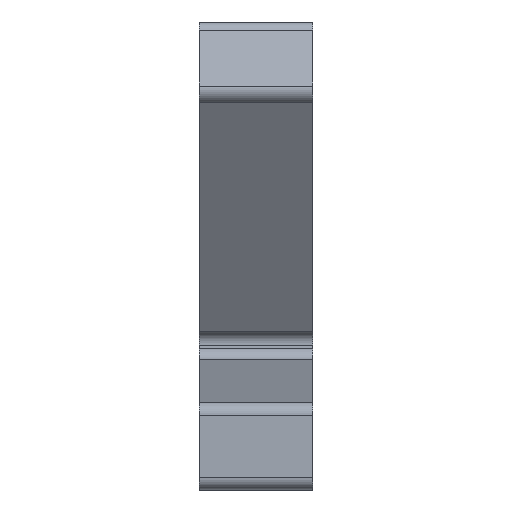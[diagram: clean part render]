
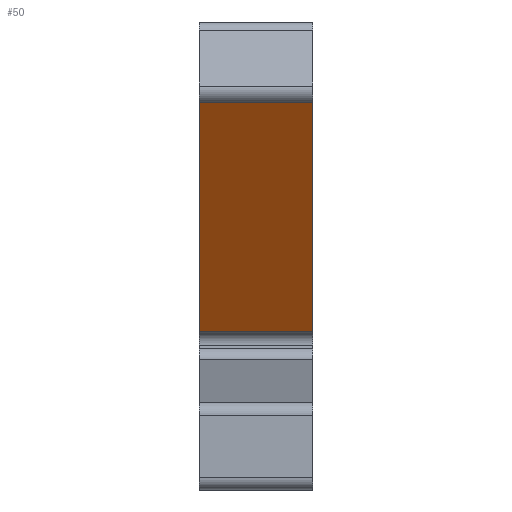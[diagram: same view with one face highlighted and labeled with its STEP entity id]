
A CAD part, left-side view. The second image highlights one B-rep face of the part: STEP entity #50.
In plain terms, the highlighted planar face has unit normal (-0.267, 0, -0.964).
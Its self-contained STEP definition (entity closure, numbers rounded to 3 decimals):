
#50 = ADVANCED_FACE ( 'NONE', ( #385 ), #720, .T. ) ;
#65 = EDGE_CURVE ( 'NONE', #340, #339, #403, .T. ) ;
#74 = EDGE_CURVE ( 'NONE', #340, #660, #394, .T. ) ;
#75 = EDGE_CURVE ( 'NONE', #342, #339, #419, .T. ) ;
#105 = AXIS2_PLACEMENT_3D ( 'NONE', #727, #778, #777 ) ;
#194 = CARTESIAN_POINT ( 'NONE',  ( 45.203, 0., 29.295 ) ) ;
#195 = CARTESIAN_POINT ( 'NONE',  ( 45.203, 9., 29.295 ) ) ;
#196 = CARTESIAN_POINT ( 'NONE',  ( 110.7, 9., 11.158 ) ) ;
#261 = CARTESIAN_POINT ( 'NONE',  ( 111.57, 9., 10.917 ) ) ;
#271 = DIRECTION ( 'NONE',  ( 0., 1., 0. ) ) ;
#272 = DIRECTION ( 'NONE',  ( 0., -1., 0. ) ) ;
#277 = CARTESIAN_POINT ( 'NONE',  ( 110.7, 0., 11.158 ) ) ;
#278 = CARTESIAN_POINT ( 'NONE',  ( 45.203, 0., 29.295 ) ) ;
#283 = DIRECTION ( 'NONE',  ( -0.964, 0., 0.267 ) ) ;
#339 = VERTEX_POINT ( 'NONE', #195 ) ;
#340 = VERTEX_POINT ( 'NONE', #196 ) ;
#342 = VERTEX_POINT ( 'NONE', #194 ) ;
#385 = FACE_OUTER_BOUND ( 'NONE', #716, .T. ) ;
#394 = LINE ( 'NONE', #277, #422 ) ;
#403 = LINE ( 'NONE', #261, #409 ) ;
#409 = VECTOR ( 'NONE', #283, 1000. ) ;
#419 = LINE ( 'NONE', #278, #424 ) ;
#422 = VECTOR ( 'NONE', #272, 1000. ) ;
#424 = VECTOR ( 'NONE', #271, 1000. ) ;
#499 = LINE ( 'NONE', #898, #501 ) ;
#501 = VECTOR ( 'NONE', #897, 1000. ) ;
#568 = ORIENTED_EDGE ( 'NONE', *, *, #75, .T. ) ;
#569 = ORIENTED_EDGE ( 'NONE', *, *, #625, .T. ) ;
#570 = ORIENTED_EDGE ( 'NONE', *, *, #74, .T. ) ;
#571 = ORIENTED_EDGE ( 'NONE', *, *, #65, .F. ) ;
#625 = EDGE_CURVE ( 'NONE', #660, #342, #499, .T. ) ;
#660 = VERTEX_POINT ( 'NONE', #827 ) ;
#716 = EDGE_LOOP ( 'NONE', ( #571, #570, #569, #568 ) ) ;
#720 = PLANE ( 'NONE',  #105 ) ;
#727 = CARTESIAN_POINT ( 'NONE',  ( 111.57, 0., 10.917 ) ) ;
#777 = DIRECTION ( 'NONE',  ( -0.964, 0., 0.267 ) ) ;
#778 = DIRECTION ( 'NONE',  ( -0.267, 0., -0.964 ) ) ;
#827 = CARTESIAN_POINT ( 'NONE',  ( 110.7, 0., 11.158 ) ) ;
#897 = DIRECTION ( 'NONE',  ( -0.964, 0., 0.267 ) ) ;
#898 = CARTESIAN_POINT ( 'NONE',  ( 111.57, 0., 10.917 ) ) ;
